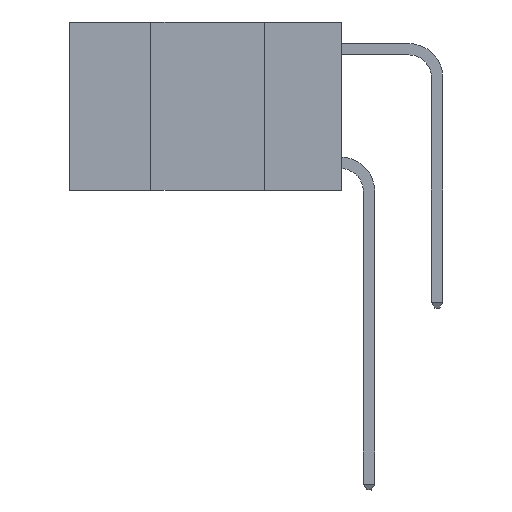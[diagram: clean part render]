
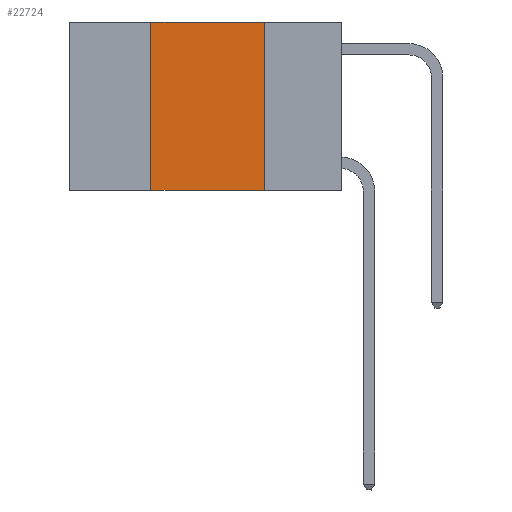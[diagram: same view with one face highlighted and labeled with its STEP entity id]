
A CAD part, left-side view. The second image highlights one B-rep face of the part: STEP entity #22724.
In plain terms, the highlighted planar face has unit normal (-1, 0, 0).
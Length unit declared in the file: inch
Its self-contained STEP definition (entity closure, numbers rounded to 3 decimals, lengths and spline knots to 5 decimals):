
#1557 = LINE ( 'NONE', #11061, #5553 ) ;
#5553 = VECTOR ( 'NONE', #12420, 39.37008 ) ;
#6726 = CARTESIAN_POINT ( 'NONE',  ( 0., 0.42, -0.37 ) ) ;
#7355 = CARTESIAN_POINT ( 'NONE',  ( 0., 0.42, 0. ) ) ;
#7790 = CARTESIAN_POINT ( 'NONE',  ( 0., 0.17, 0. ) ) ;
#8721 = LINE ( 'NONE', #26262, #15609 ) ;
#8846 = LINE ( 'NONE', #15946, #9599 ) ;
#9322 = VERTEX_POINT ( 'NONE', #7790 ) ;
#9599 = VECTOR ( 'NONE', #14031, 39.37008 ) ;
#9689 = VERTEX_POINT ( 'NONE', #6726 ) ;
#11061 = CARTESIAN_POINT ( 'NONE',  ( 0., 0.42, 0. ) ) ;
#12347 = EDGE_CURVE ( 'NONE', #15267, #9322, #19683, .T. ) ;
#12420 = DIRECTION ( 'NONE',  ( 0., 0., 1. ) ) ;
#13823 = EDGE_LOOP ( 'NONE', ( #23282, #13841, #20052, #21572 ) ) ;
#13841 = ORIENTED_EDGE ( 'NONE', *, *, #12347, .F. ) ;
#14031 = DIRECTION ( 'NONE',  ( 0., 0., -1. ) ) ;
#14822 = DIRECTION ( 'NONE',  ( 0., -1., 0. ) ) ;
#15267 = VERTEX_POINT ( 'NONE', #7355 ) ;
#15297 = AXIS2_PLACEMENT_3D ( 'NONE', #23064, #27896, #25284 ) ;
#15609 = VECTOR ( 'NONE', #19920, 39.37008 ) ;
#15946 = CARTESIAN_POINT ( 'NONE',  ( 0., 0.17, 0. ) ) ;
#15960 = PLANE ( 'NONE',  #15297 ) ;
#16445 = FACE_OUTER_BOUND ( 'NONE', #13823, .T. ) ;
#17365 = VERTEX_POINT ( 'NONE', #28846 ) ;
#18977 = EDGE_CURVE ( 'NONE', #9322, #17365, #8846, .T. ) ;
#19683 = LINE ( 'NONE', #23243, #25904 ) ;
#19920 = DIRECTION ( 'NONE',  ( 0., -1., 0. ) ) ;
#20052 = ORIENTED_EDGE ( 'NONE', *, *, #20462, .F. ) ;
#20462 = EDGE_CURVE ( 'NONE', #9689, #15267, #1557, .T. ) ;
#21572 = ORIENTED_EDGE ( 'NONE', *, *, #25850, .T. ) ;
#22724 = ADVANCED_FACE ( 'NONE', ( #16445 ), #15960, .F. ) ;
#23064 = CARTESIAN_POINT ( 'NONE',  ( 0., 0.6, 0. ) ) ;
#23243 = CARTESIAN_POINT ( 'NONE',  ( 0., 0.6, 0. ) ) ;
#23282 = ORIENTED_EDGE ( 'NONE', *, *, #18977, .F. ) ;
#25284 = DIRECTION ( 'NONE',  ( 0., 0., -1. ) ) ;
#25850 = EDGE_CURVE ( 'NONE', #9689, #17365, #8721, .T. ) ;
#25904 = VECTOR ( 'NONE', #14822, 39.37008 ) ;
#26262 = CARTESIAN_POINT ( 'NONE',  ( 0., 0.6, -0.37 ) ) ;
#27896 = DIRECTION ( 'NONE',  ( 1., 0., 0. ) ) ;
#28846 = CARTESIAN_POINT ( 'NONE',  ( 0., 0.17, -0.37 ) ) ;
